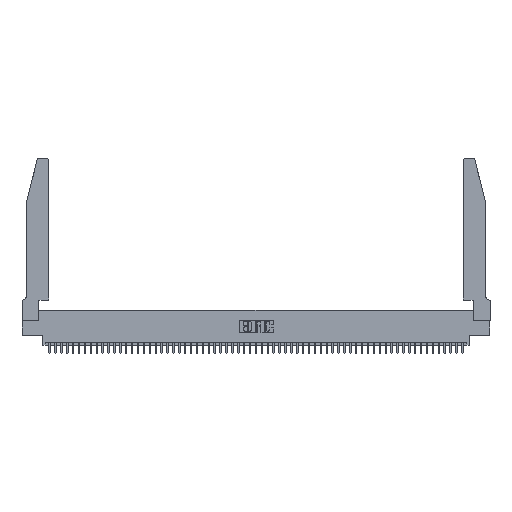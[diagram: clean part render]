
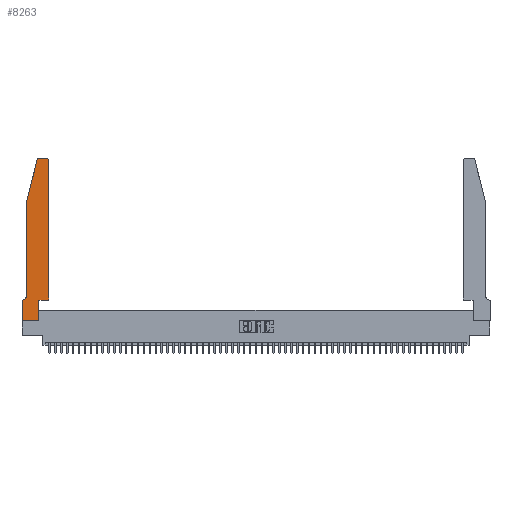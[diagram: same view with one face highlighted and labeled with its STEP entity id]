
A CAD part, top view. The second image highlights one B-rep face of the part: STEP entity #8263.
In plain terms, the highlighted planar face has unit normal (0, 0, 1).
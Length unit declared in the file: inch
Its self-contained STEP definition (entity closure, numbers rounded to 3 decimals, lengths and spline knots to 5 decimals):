
#550 = CARTESIAN_POINT ( 'NONE',  ( 0.0755, 2., 0.37 ) ) ;
#3904 = VERTEX_POINT ( 'NONE', #9591 ) ;
#5037 = DIRECTION ( 'NONE',  ( 0., -1., 0. ) ) ;
#6012 = FACE_OUTER_BOUND ( 'NONE', #32653, .T. ) ;
#6405 = CARTESIAN_POINT ( 'NONE',  ( 0.4205, 2.75, 0.37 ) ) ;
#6659 = EDGE_CURVE ( 'NONE', #7927, #38037, #18600, .T. ) ;
#6825 = DIRECTION ( 'NONE',  ( 0., 0., 1. ) ) ;
#7927 = VERTEX_POINT ( 'NONE', #43145 ) ;
#8263 = ADVANCED_FACE ( 'NONE', ( #6012 ), #41598, .T. ) ;
#9591 = CARTESIAN_POINT ( 'NONE',  ( 0.2865, 0.35, 0.37 ) ) ;
#9946 = EDGE_CURVE ( 'NONE', #3904, #7927, #56438, .T. ) ;
#11155 = CARTESIAN_POINT ( 'NONE',  ( 0.2865, 0.35, 0.37 ) ) ;
#11969 = VERTEX_POINT ( 'NONE', #17545 ) ;
#12041 = LINE ( 'NONE', #26708, #33989 ) ;
#12160 = VERTEX_POINT ( 'NONE', #32067 ) ;
#12613 = LINE ( 'NONE', #16455, #44730 ) ;
#13691 = DIRECTION ( 'NONE',  ( 1., 0., 0. ) ) ;
#15326 = AXIS2_PLACEMENT_3D ( 'NONE', #43698, #17539, #48062 ) ;
#15845 = VECTOR ( 'NONE', #56542, 39.37008 ) ;
#16455 = CARTESIAN_POINT ( 'NONE',  ( 0.0755, 0.35, 0.37 ) ) ;
#16825 = EDGE_CURVE ( 'NONE', #21233, #41548, #19660, .T. ) ;
#17043 = AXIS2_PLACEMENT_3D ( 'NONE', #33110, #6825, #37494 ) ;
#17117 = CARTESIAN_POINT ( 'NONE',  ( 0., 0., 0.37 ) ) ;
#17179 = EDGE_CURVE ( 'NONE', #31733, #32062, #12041, .T. ) ;
#17539 = DIRECTION ( 'NONE',  ( 0., 0., 1. ) ) ;
#17545 = CARTESIAN_POINT ( 'NONE',  ( 0.2865, 0., 0.37 ) ) ;
#18170 = CARTESIAN_POINT ( 'NONE',  ( 0., 0., 0.37 ) ) ;
#18334 = EDGE_CURVE ( 'NONE', #41548, #31733, #12613, .T. ) ;
#18600 = LINE ( 'NONE', #30215, #50665 ) ;
#19660 = CIRCLE ( 'NONE', #33543, 0.07 ) ;
#19832 = DIRECTION ( 'NONE',  ( 1., 0., 0. ) ) ;
#21233 = VERTEX_POINT ( 'NONE', #44215 ) ;
#21643 = VECTOR ( 'NONE', #13691, 39.37008 ) ;
#22639 = EDGE_CURVE ( 'NONE', #11969, #3904, #56621, .T. ) ;
#23495 = CARTESIAN_POINT ( 'NONE',  ( 0.0055, 0.42, 0.37 ) ) ;
#23814 = VERTEX_POINT ( 'NONE', #6405 ) ;
#23855 = ORIENTED_EDGE ( 'NONE', *, *, #40735, .T. ) ;
#24308 = VECTOR ( 'NONE', #38877, 39.37008 ) ;
#24423 = DIRECTION ( 'NONE',  ( -1., 0., 0. ) ) ;
#24870 = EDGE_CURVE ( 'NONE', #32062, #11969, #38638, .T. ) ;
#25064 = CARTESIAN_POINT ( 'NONE',  ( 0.4505, 2.72, 0.37 ) ) ;
#26038 = ORIENTED_EDGE ( 'NONE', *, *, #40514, .T. ) ;
#26371 = AXIS2_PLACEMENT_3D ( 'NONE', #50138, #45940, #19832 ) ;
#26580 = ORIENTED_EDGE ( 'NONE', *, *, #42677, .T. ) ;
#26708 = CARTESIAN_POINT ( 'NONE',  ( 0., 0., 0.37 ) ) ;
#27886 = DIRECTION ( 'NONE',  ( -1., 0., 0. ) ) ;
#28877 = LINE ( 'NONE', #38813, #15845 ) ;
#29283 = CARTESIAN_POINT ( 'NONE',  ( 0.284, 2.75, 0.37 ) ) ;
#29481 = CIRCLE ( 'NONE', #15326, 0.03 ) ;
#30215 = CARTESIAN_POINT ( 'NONE',  ( 0.4505, 0.35, 0.37 ) ) ;
#30302 = CARTESIAN_POINT ( 'NONE',  ( 0.0755, 2., 0.37 ) ) ;
#30413 = VECTOR ( 'NONE', #24423, 39.37008 ) ;
#31733 = VERTEX_POINT ( 'NONE', #32524 ) ;
#32062 = VERTEX_POINT ( 'NONE', #18170 ) ;
#32067 = CARTESIAN_POINT ( 'NONE',  ( 0.25487, 2.72718, 0.37 ) ) ;
#32425 = VECTOR ( 'NONE', #5037, 39.37008 ) ;
#32524 = CARTESIAN_POINT ( 'NONE',  ( 0., 0.35, 0.37 ) ) ;
#32653 = EDGE_LOOP ( 'NONE', ( #26038, #26580, #37458, #23855, #48983, #39810, #54207, #44940, #34968, #36865, #49081, #49807 ) ) ;
#33110 = CARTESIAN_POINT ( 'NONE',  ( 0.4205, 2.72, 0.37 ) ) ;
#33543 = AXIS2_PLACEMENT_3D ( 'NONE', #23495, #53979, #27886 ) ;
#33989 = VECTOR ( 'NONE', #52794, 39.37008 ) ;
#34968 = ORIENTED_EDGE ( 'NONE', *, *, #22639, .T. ) ;
#36393 = CARTESIAN_POINT ( 'NONE',  ( 0.0055, 0.35, 0.37 ) ) ;
#36865 = ORIENTED_EDGE ( 'NONE', *, *, #9946, .T. ) ;
#37458 = ORIENTED_EDGE ( 'NONE', *, *, #42006, .T. ) ;
#37494 = DIRECTION ( 'NONE',  ( 1., 0., 0. ) ) ;
#38037 = VERTEX_POINT ( 'NONE', #25064 ) ;
#38411 = DIRECTION ( 'NONE',  ( -1., 0., 0. ) ) ;
#38638 = LINE ( 'NONE', #17117, #24308 ) ;
#38813 = CARTESIAN_POINT ( 'NONE',  ( 0.0755, 2., 0.37 ) ) ;
#38877 = DIRECTION ( 'NONE',  ( 1., 0., 0. ) ) ;
#39810 = ORIENTED_EDGE ( 'NONE', *, *, #18334, .T. ) ;
#39944 = CIRCLE ( 'NONE', #17043, 0.03 ) ;
#40514 = EDGE_CURVE ( 'NONE', #23814, #47294, #53565, .T. ) ;
#40735 = EDGE_CURVE ( 'NONE', #46777, #21233, #55592, .T. ) ;
#41548 = VERTEX_POINT ( 'NONE', #36393 ) ;
#41598 = PLANE ( 'NONE',  #26371 ) ;
#42006 = EDGE_CURVE ( 'NONE', #12160, #46777, #28877, .T. ) ;
#42677 = EDGE_CURVE ( 'NONE', #47294, #12160, #29481, .T. ) ;
#43145 = CARTESIAN_POINT ( 'NONE',  ( 0.4505, 0.35, 0.37 ) ) ;
#43698 = CARTESIAN_POINT ( 'NONE',  ( 0.284, 2.72, 0.37 ) ) ;
#44215 = CARTESIAN_POINT ( 'NONE',  ( 0.0755, 0.42, 0.37 ) ) ;
#44730 = VECTOR ( 'NONE', #38411, 39.37008 ) ;
#44940 = ORIENTED_EDGE ( 'NONE', *, *, #24870, .T. ) ;
#45006 = VECTOR ( 'NONE', #54876, 39.37008 ) ;
#45940 = DIRECTION ( 'NONE',  ( 0., 0., 1. ) ) ;
#46777 = VERTEX_POINT ( 'NONE', #30302 ) ;
#47294 = VERTEX_POINT ( 'NONE', #29283 ) ;
#48062 = DIRECTION ( 'NONE',  ( 1., 0., 0. ) ) ;
#48983 = ORIENTED_EDGE ( 'NONE', *, *, #16825, .T. ) ;
#49056 = EDGE_CURVE ( 'NONE', #38037, #23814, #39944, .T. ) ;
#49081 = ORIENTED_EDGE ( 'NONE', *, *, #6659, .T. ) ;
#49807 = ORIENTED_EDGE ( 'NONE', *, *, #49056, .T. ) ;
#50138 = CARTESIAN_POINT ( 'NONE',  ( 0., 0.35, 0.37 ) ) ;
#50518 = CARTESIAN_POINT ( 'NONE',  ( 0.2605, 2.75, 0.37 ) ) ;
#50665 = VECTOR ( 'NONE', #51894, 39.37008 ) ;
#51894 = DIRECTION ( 'NONE',  ( 0., 1., 0. ) ) ;
#52794 = DIRECTION ( 'NONE',  ( 0., -1., 0. ) ) ;
#52818 = CARTESIAN_POINT ( 'NONE',  ( 0.4505, 0.35, 0.37 ) ) ;
#53565 = LINE ( 'NONE', #50518, #30413 ) ;
#53979 = DIRECTION ( 'NONE',  ( 0., 0., -1. ) ) ;
#54207 = ORIENTED_EDGE ( 'NONE', *, *, #17179, .T. ) ;
#54876 = DIRECTION ( 'NONE',  ( 0., 1., 0. ) ) ;
#55592 = LINE ( 'NONE', #550, #32425 ) ;
#56438 = LINE ( 'NONE', #52818, #21643 ) ;
#56542 = DIRECTION ( 'NONE',  ( -0.239, -0.971, 0. ) ) ;
#56621 = LINE ( 'NONE', #11155, #45006 ) ;
